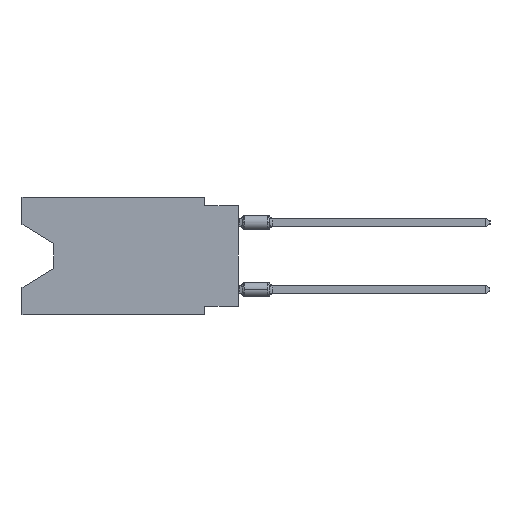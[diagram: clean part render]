
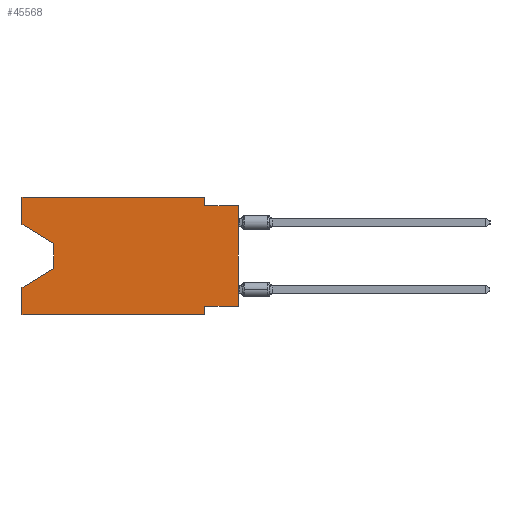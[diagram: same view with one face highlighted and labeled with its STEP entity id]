
A CAD part, left-side view. The second image highlights one B-rep face of the part: STEP entity #45568.
In plain terms, the highlighted planar face has unit normal (-1, 0, 0).
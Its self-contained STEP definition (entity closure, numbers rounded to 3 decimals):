
#582 = ORIENTED_EDGE ( 'NONE', *, *, #17537, .T. ) ;
#1293 = EDGE_CURVE ( 'NONE', #41103, #46934, #19563, .T. ) ;
#2042 = VECTOR ( 'NONE', #28230, 1000. ) ;
#2133 = VECTOR ( 'NONE', #16147, 1000. ) ;
#2237 = LINE ( 'NONE', #12654, #16256 ) ;
#2478 = DIRECTION ( 'NONE',  ( 0., 0., -1. ) ) ;
#2519 = VERTEX_POINT ( 'NONE', #29882 ) ;
#2946 = EDGE_CURVE ( 'NONE', #35211, #31920, #12428, .T. ) ;
#3053 = PLANE ( 'NONE',  #37383 ) ;
#3068 = EDGE_CURVE ( 'NONE', #42051, #40856, #42448, .T. ) ;
#3334 = CARTESIAN_POINT ( 'NONE',  ( 0., 16.383, -6.852 ) ) ;
#4487 = ORIENTED_EDGE ( 'NONE', *, *, #2946, .T. ) ;
#5062 = CARTESIAN_POINT ( 'NONE',  ( 0., 13.97, -3.505 ) ) ;
#5115 = VERTEX_POINT ( 'NONE', #22369 ) ;
#5840 = ORIENTED_EDGE ( 'NONE', *, *, #34112, .F. ) ;
#6265 = LINE ( 'NONE', #49467, #45111 ) ;
#7348 = FACE_OUTER_BOUND ( 'NONE', #33229, .T. ) ;
#7477 = VERTEX_POINT ( 'NONE', #37707 ) ;
#7652 = EDGE_CURVE ( 'NONE', #38815, #35211, #8868, .T. ) ;
#7898 = ORIENTED_EDGE ( 'NONE', *, *, #1293, .F. ) ;
#8018 = CARTESIAN_POINT ( 'NONE',  ( 0., 2.54, -8.89 ) ) ;
#8264 = CARTESIAN_POINT ( 'NONE',  ( 0., 16.383, 0. ) ) ;
#8521 = CARTESIAN_POINT ( 'NONE',  ( 0., 2.54, -8.255 ) ) ;
#8868 = LINE ( 'NONE', #5062, #22941 ) ;
#10021 = LINE ( 'NONE', #41112, #45967 ) ;
#11130 = LINE ( 'NONE', #18724, #11840 ) ;
#11840 = VECTOR ( 'NONE', #38928, 1000. ) ;
#12428 = LINE ( 'NONE', #27847, #49400 ) ;
#12654 = CARTESIAN_POINT ( 'NONE',  ( 0., 0., 0. ) ) ;
#14013 = VECTOR ( 'NONE', #24908, 1000. ) ;
#14453 = EDGE_CURVE ( 'NONE', #7477, #21368, #10021, .T. ) ;
#15155 = ORIENTED_EDGE ( 'NONE', *, *, #14453, .F. ) ;
#15158 = CARTESIAN_POINT ( 'NONE',  ( 0., 2.54, -8.89 ) ) ;
#15392 = VECTOR ( 'NONE', #47636, 1000. ) ;
#16009 = EDGE_CURVE ( 'NONE', #48384, #46934, #2237, .T. ) ;
#16147 = DIRECTION ( 'NONE',  ( 0., -0.855, -0.519 ) ) ;
#16256 = VECTOR ( 'NONE', #43477, 1000. ) ;
#16808 = CARTESIAN_POINT ( 'NONE',  ( 0., 0., -8.255 ) ) ;
#17451 = DIRECTION ( 'NONE',  ( 0., 0.855, -0.519 ) ) ;
#17537 = EDGE_CURVE ( 'NONE', #7477, #38815, #46972, .T. ) ;
#18467 = ORIENTED_EDGE ( 'NONE', *, *, #3068, .F. ) ;
#18724 = CARTESIAN_POINT ( 'NONE',  ( 0., 16.383, 0. ) ) ;
#18827 = CARTESIAN_POINT ( 'NONE',  ( 0., 2.54, -0.635 ) ) ;
#19075 = DIRECTION ( 'NONE',  ( 0., -1., 0. ) ) ;
#19563 = LINE ( 'NONE', #30945, #30128 ) ;
#21025 = CARTESIAN_POINT ( 'NONE',  ( 0., 13.97, -3.505 ) ) ;
#21045 = CARTESIAN_POINT ( 'NONE',  ( 0., 0., -8.255 ) ) ;
#21110 = CARTESIAN_POINT ( 'NONE',  ( 0., 16.383, -8.89 ) ) ;
#21368 = VERTEX_POINT ( 'NONE', #44200 ) ;
#21911 = DIRECTION ( 'NONE',  ( 0., 0., 1. ) ) ;
#22369 = CARTESIAN_POINT ( 'NONE',  ( 0., 16.383, -8.89 ) ) ;
#22941 = VECTOR ( 'NONE', #35907, 1000. ) ;
#23823 = EDGE_CURVE ( 'NONE', #48384, #42051, #28669, .T. ) ;
#24908 = DIRECTION ( 'NONE',  ( 0., -1., 0. ) ) ;
#25727 = EDGE_CURVE ( 'NONE', #5115, #40856, #28448, .T. ) ;
#26308 = DIRECTION ( 'NONE',  ( 0., 0., -1. ) ) ;
#27847 = CARTESIAN_POINT ( 'NONE',  ( 0., 13.97, -5.385 ) ) ;
#27992 = LINE ( 'NONE', #8264, #2042 ) ;
#28230 = DIRECTION ( 'NONE',  ( 0., 0., 1. ) ) ;
#28448 = LINE ( 'NONE', #21110, #14013 ) ;
#28669 = LINE ( 'NONE', #16808, #15392 ) ;
#29772 = CARTESIAN_POINT ( 'NONE',  ( 0., 13.97, -5.385 ) ) ;
#29882 = CARTESIAN_POINT ( 'NONE',  ( 0., 2.54, 0. ) ) ;
#30128 = VECTOR ( 'NONE', #19075, 1000. ) ;
#30945 = CARTESIAN_POINT ( 'NONE',  ( 0., 0., -0.635 ) ) ;
#31920 = VERTEX_POINT ( 'NONE', #3334 ) ;
#32465 = ORIENTED_EDGE ( 'NONE', *, *, #23823, .F. ) ;
#33229 = EDGE_LOOP ( 'NONE', ( #582, #48534, #4487, #5840, #49436, #18467, #32465, #47076, #7898, #40508, #33540, #15155 ) ) ;
#33540 = ORIENTED_EDGE ( 'NONE', *, *, #43300, .F. ) ;
#34112 = EDGE_CURVE ( 'NONE', #5115, #31920, #27992, .T. ) ;
#34145 = DIRECTION ( 'NONE',  ( 1., 0., 0. ) ) ;
#34850 = CARTESIAN_POINT ( 'NONE',  ( 0., 16.383, -2.038 ) ) ;
#35211 = VERTEX_POINT ( 'NONE', #29772 ) ;
#35907 = DIRECTION ( 'NONE',  ( 0., 0., -1. ) ) ;
#36397 = CARTESIAN_POINT ( 'NONE',  ( 0., 0., -0.635 ) ) ;
#37383 = AXIS2_PLACEMENT_3D ( 'NONE', #37431, #34145, #26308 ) ;
#37431 = CARTESIAN_POINT ( 'NONE',  ( 0., 16.383, 0. ) ) ;
#37707 = CARTESIAN_POINT ( 'NONE',  ( 0., 16.383, -2.038 ) ) ;
#37910 = DIRECTION ( 'NONE',  ( 0., 0., -1. ) ) ;
#38815 = VERTEX_POINT ( 'NONE', #21025 ) ;
#38928 = DIRECTION ( 'NONE',  ( 0., -1., 0. ) ) ;
#40508 = ORIENTED_EDGE ( 'NONE', *, *, #40634, .F. ) ;
#40634 = EDGE_CURVE ( 'NONE', #2519, #41103, #6265, .T. ) ;
#40856 = VERTEX_POINT ( 'NONE', #8018 ) ;
#41103 = VERTEX_POINT ( 'NONE', #18827 ) ;
#41112 = CARTESIAN_POINT ( 'NONE',  ( 0., 16.383, 0. ) ) ;
#42051 = VERTEX_POINT ( 'NONE', #8521 ) ;
#42448 = LINE ( 'NONE', #15158, #47737 ) ;
#43300 = EDGE_CURVE ( 'NONE', #21368, #2519, #11130, .T. ) ;
#43477 = DIRECTION ( 'NONE',  ( 0., 0., 1. ) ) ;
#44200 = CARTESIAN_POINT ( 'NONE',  ( 0., 16.383, 0. ) ) ;
#45111 = VECTOR ( 'NONE', #2478, 1000. ) ;
#45568 = ADVANCED_FACE ( 'NONE', ( #7348 ), #3053, .F. ) ;
#45967 = VECTOR ( 'NONE', #21911, 1000. ) ;
#46934 = VERTEX_POINT ( 'NONE', #36397 ) ;
#46972 = LINE ( 'NONE', #34850, #2133 ) ;
#47076 = ORIENTED_EDGE ( 'NONE', *, *, #16009, .T. ) ;
#47636 = DIRECTION ( 'NONE',  ( 0., 1., 0. ) ) ;
#47737 = VECTOR ( 'NONE', #37910, 1000. ) ;
#48384 = VERTEX_POINT ( 'NONE', #21045 ) ;
#48534 = ORIENTED_EDGE ( 'NONE', *, *, #7652, .T. ) ;
#49400 = VECTOR ( 'NONE', #17451, 1000. ) ;
#49436 = ORIENTED_EDGE ( 'NONE', *, *, #25727, .T. ) ;
#49467 = CARTESIAN_POINT ( 'NONE',  ( 0., 2.54, 0. ) ) ;
